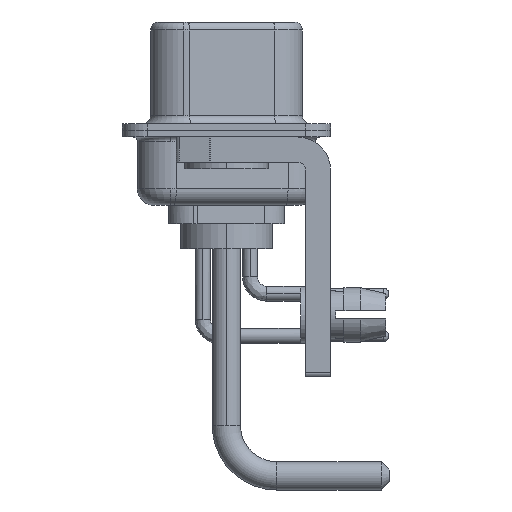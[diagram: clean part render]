
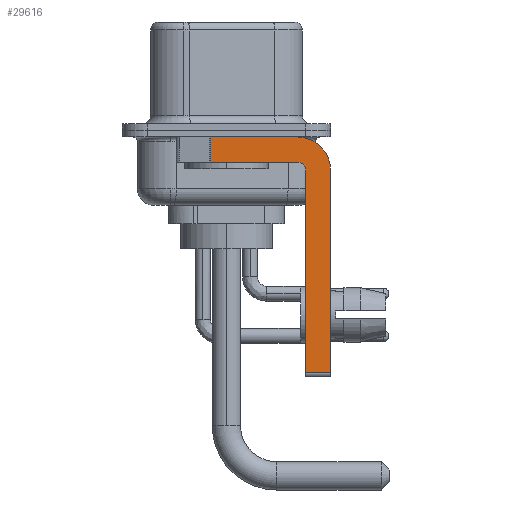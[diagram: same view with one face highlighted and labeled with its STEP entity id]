
A CAD part, left-side view. The second image highlights one B-rep face of the part: STEP entity #29616.
In plain terms, the highlighted planar face has unit normal (-1, 0, 0).
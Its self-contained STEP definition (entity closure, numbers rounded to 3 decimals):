
#848 = DIRECTION ( 'NONE',  ( 0., 0., -1. ) ) ;
#1299 = LINE ( 'NONE', #8049, #13883 ) ;
#1352 = CIRCLE ( 'NONE', #15092, 2. ) ;
#2035 = VECTOR ( 'NONE', #27459, 1000. ) ;
#2092 = CARTESIAN_POINT ( 'NONE',  ( -2.9, -4.25, -0.4 ) ) ;
#2235 = ORIENTED_EDGE ( 'NONE', *, *, #25780, .F. ) ;
#2704 = VERTEX_POINT ( 'NONE', #13568 ) ;
#3849 = VECTOR ( 'NONE', #13807, 1000. ) ;
#4907 = VERTEX_POINT ( 'NONE', #23438 ) ;
#4978 = EDGE_LOOP ( 'NONE', ( #7013, #25859, #5110, #7570, #2235, #13780, #22471, #20891 ) ) ;
#5110 = ORIENTED_EDGE ( 'NONE', *, *, #21999, .F. ) ;
#6174 = CARTESIAN_POINT ( 'NONE',  ( -2.9, -4.25, -2.4 ) ) ;
#6677 = EDGE_CURVE ( 'NONE', #17425, #4907, #1299, .T. ) ;
#7013 = ORIENTED_EDGE ( 'NONE', *, *, #27704, .F. ) ;
#7033 = VECTOR ( 'NONE', #15279, 1000. ) ;
#7570 = ORIENTED_EDGE ( 'NONE', *, *, #25624, .F. ) ;
#8049 = CARTESIAN_POINT ( 'NONE',  ( -2.9, -6.25, -2.4 ) ) ;
#9000 = DIRECTION ( 'NONE',  ( 1., 0., 0. ) ) ;
#9749 = VECTOR ( 'NONE', #29502, 1000. ) ;
#11291 = VERTEX_POINT ( 'NONE', #24049 ) ;
#11354 = CARTESIAN_POINT ( 'NONE',  ( -2.9, -4.25, -14.55 ) ) ;
#11659 = CARTESIAN_POINT ( 'NONE',  ( -2.9, 3., -0.4 ) ) ;
#13492 = CARTESIAN_POINT ( 'NONE',  ( -2.9, -4.25, -1.9 ) ) ;
#13568 = CARTESIAN_POINT ( 'NONE',  ( -2.9, -4.75, -14.55 ) ) ;
#13780 = ORIENTED_EDGE ( 'NONE', *, *, #28477, .T. ) ;
#13807 = DIRECTION ( 'NONE',  ( 0., 1., 0. ) ) ;
#13883 = VECTOR ( 'NONE', #848, 1000. ) ;
#14647 = DIRECTION ( 'NONE',  ( -1., 0., 0. ) ) ;
#15092 = AXIS2_PLACEMENT_3D ( 'NONE', #16369, #9000, #20813 ) ;
#15279 = DIRECTION ( 'NONE',  ( 0., 0., -1. ) ) ;
#15397 = LINE ( 'NONE', #18163, #9749 ) ;
#15547 = FACE_OUTER_BOUND ( 'NONE', #4978, .T. ) ;
#15971 = DIRECTION ( 'NONE',  ( 0., -1., 0. ) ) ;
#16012 = PLANE ( 'NONE',  #25522 ) ;
#16369 = CARTESIAN_POINT ( 'NONE',  ( -2.9, -4.25, -2.4 ) ) ;
#16410 = VERTEX_POINT ( 'NONE', #19259 ) ;
#17425 = VERTEX_POINT ( 'NONE', #26976 ) ;
#17912 = EDGE_CURVE ( 'NONE', #26205, #18112, #29071, .T. ) ;
#18112 = VERTEX_POINT ( 'NONE', #25380 ) ;
#18163 = CARTESIAN_POINT ( 'NONE',  ( -2.9, -4.75, -14.8 ) ) ;
#19067 = AXIS2_PLACEMENT_3D ( 'NONE', #19397, #14647, #24434 ) ;
#19259 = CARTESIAN_POINT ( 'NONE',  ( -2.9, -4.75, -2.4 ) ) ;
#19397 = CARTESIAN_POINT ( 'NONE',  ( -2.9, -4.25, -2.4 ) ) ;
#20177 = VERTEX_POINT ( 'NONE', #2092 ) ;
#20200 = EDGE_CURVE ( 'NONE', #20177, #17425, #1352, .T. ) ;
#20813 = DIRECTION ( 'NONE',  ( 0., 0., -1. ) ) ;
#20891 = ORIENTED_EDGE ( 'NONE', *, *, #20200, .F. ) ;
#21999 = EDGE_CURVE ( 'NONE', #11291, #18112, #27755, .T. ) ;
#22471 = ORIENTED_EDGE ( 'NONE', *, *, #6677, .F. ) ;
#22841 = LINE ( 'NONE', #11354, #2035 ) ;
#23438 = CARTESIAN_POINT ( 'NONE',  ( -2.9, -6.25, -14.55 ) ) ;
#23543 = VECTOR ( 'NONE', #15971, 1000. ) ;
#24049 = CARTESIAN_POINT ( 'NONE',  ( -2.9, -4.25, -1.9 ) ) ;
#24434 = DIRECTION ( 'NONE',  ( 0., 0., 1. ) ) ;
#24740 = DIRECTION ( 'NONE',  ( 0., 0., -1. ) ) ;
#25380 = CARTESIAN_POINT ( 'NONE',  ( -2.9, 0.978, -1.9 ) ) ;
#25419 = CIRCLE ( 'NONE', #19067, 0.5 ) ;
#25522 = AXIS2_PLACEMENT_3D ( 'NONE', #6174, #29793, #24740 ) ;
#25624 = EDGE_CURVE ( 'NONE', #16410, #11291, #25419, .T. ) ;
#25752 = LINE ( 'NONE', #11659, #23543 ) ;
#25780 = EDGE_CURVE ( 'NONE', #2704, #16410, #15397, .T. ) ;
#25859 = ORIENTED_EDGE ( 'NONE', *, *, #17912, .T. ) ;
#26205 = VERTEX_POINT ( 'NONE', #27738 ) ;
#26611 = CARTESIAN_POINT ( 'NONE',  ( -2.9, 0.978, -1.9 ) ) ;
#26976 = CARTESIAN_POINT ( 'NONE',  ( -2.9, -6.25, -2.4 ) ) ;
#27459 = DIRECTION ( 'NONE',  ( 0., -1., 0. ) ) ;
#27704 = EDGE_CURVE ( 'NONE', #26205, #20177, #25752, .T. ) ;
#27738 = CARTESIAN_POINT ( 'NONE',  ( -2.9, 0.978, -0.4 ) ) ;
#27755 = LINE ( 'NONE', #13492, #3849 ) ;
#28477 = EDGE_CURVE ( 'NONE', #2704, #4907, #22841, .T. ) ;
#29071 = LINE ( 'NONE', #26611, #7033 ) ;
#29502 = DIRECTION ( 'NONE',  ( 0., 0., 1. ) ) ;
#29616 = ADVANCED_FACE ( 'NONE', ( #15547 ), #16012, .F. ) ;
#29793 = DIRECTION ( 'NONE',  ( 1., 0., 0. ) ) ;
